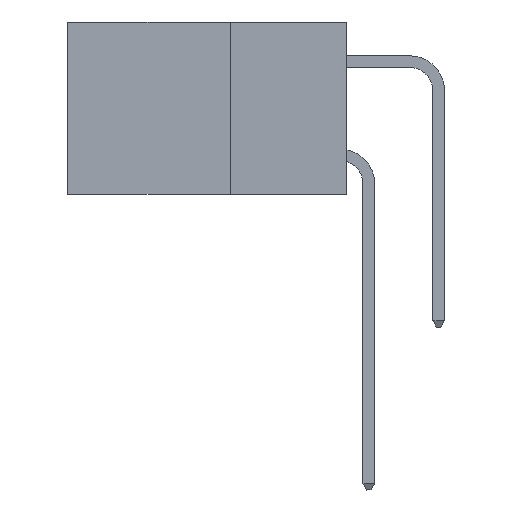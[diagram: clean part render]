
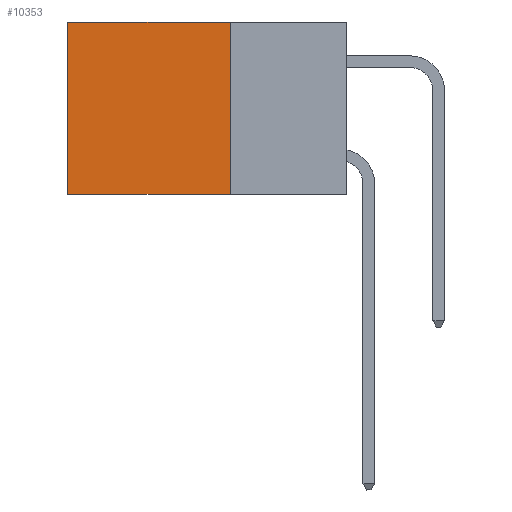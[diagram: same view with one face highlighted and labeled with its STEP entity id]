
A CAD part, left-side view. The second image highlights one B-rep face of the part: STEP entity #10353.
In plain terms, the highlighted planar face has unit normal (-1, 0, 0).
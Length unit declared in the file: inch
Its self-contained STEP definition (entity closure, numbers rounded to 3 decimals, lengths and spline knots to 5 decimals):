
#384 = LINE ( 'NONE', #24766, #29024 ) ;
#1726 = DIRECTION ( 'NONE',  ( 0., 1., 0. ) ) ;
#5333 = EDGE_CURVE ( 'NONE', #7010, #21526, #384, .T. ) ;
#6901 = CARTESIAN_POINT ( 'NONE',  ( 0.2875, 0.25, 0. ) ) ;
#7010 = VERTEX_POINT ( 'NONE', #28568 ) ;
#9095 = AXIS2_PLACEMENT_3D ( 'NONE', #33037, #10491, #24911 ) ;
#9684 = LINE ( 'NONE', #32237, #28303 ) ;
#10353 = ADVANCED_FACE ( 'NONE', ( #11183 ), #10658, .F. ) ;
#10491 = DIRECTION ( 'NONE',  ( 1., 0., 0. ) ) ;
#10658 = PLANE ( 'NONE',  #9095 ) ;
#11183 = FACE_OUTER_BOUND ( 'NONE', #15606, .T. ) ;
#12025 = CARTESIAN_POINT ( 'NONE',  ( 0.2875, 0.25, 0. ) ) ;
#12202 = CARTESIAN_POINT ( 'NONE',  ( 0.2875, 0.25, -0.37 ) ) ;
#12311 = DIRECTION ( 'NONE',  ( 0., 0., -1. ) ) ;
#12540 = VERTEX_POINT ( 'NONE', #12025 ) ;
#13928 = VERTEX_POINT ( 'NONE', #12202 ) ;
#14696 = VECTOR ( 'NONE', #12311, 39.37008 ) ;
#15580 = EDGE_CURVE ( 'NONE', #12540, #13928, #20804, .T. ) ;
#15606 = EDGE_LOOP ( 'NONE', ( #22739, #34669, #29979, #29397 ) ) ;
#17326 = VECTOR ( 'NONE', #19496, 39.37008 ) ;
#19496 = DIRECTION ( 'NONE',  ( 0., 1., 0. ) ) ;
#19716 = CARTESIAN_POINT ( 'NONE',  ( 0.2875, 0.6, -0.37 ) ) ;
#20804 = LINE ( 'NONE', #6901, #14696 ) ;
#21526 = VERTEX_POINT ( 'NONE', #19716 ) ;
#22054 = DIRECTION ( 'NONE',  ( 0., 0., -1. ) ) ;
#22739 = ORIENTED_EDGE ( 'NONE', *, *, #5333, .T. ) ;
#23210 = EDGE_CURVE ( 'NONE', #12540, #7010, #30872, .T. ) ;
#24766 = CARTESIAN_POINT ( 'NONE',  ( 0.2875, 0.6, 0. ) ) ;
#24911 = DIRECTION ( 'NONE',  ( 0., 0., -1. ) ) ;
#25100 = CARTESIAN_POINT ( 'NONE',  ( 0.2875, 0.25, 0. ) ) ;
#25356 = EDGE_CURVE ( 'NONE', #13928, #21526, #9684, .T. ) ;
#28303 = VECTOR ( 'NONE', #1726, 39.37008 ) ;
#28568 = CARTESIAN_POINT ( 'NONE',  ( 0.2875, 0.6, 0. ) ) ;
#29024 = VECTOR ( 'NONE', #22054, 39.37008 ) ;
#29397 = ORIENTED_EDGE ( 'NONE', *, *, #23210, .T. ) ;
#29979 = ORIENTED_EDGE ( 'NONE', *, *, #15580, .F. ) ;
#30872 = LINE ( 'NONE', #25100, #17326 ) ;
#32237 = CARTESIAN_POINT ( 'NONE',  ( 0.2875, 0.25, -0.37 ) ) ;
#33037 = CARTESIAN_POINT ( 'NONE',  ( 0.2875, 0.25, 0. ) ) ;
#34669 = ORIENTED_EDGE ( 'NONE', *, *, #25356, .F. ) ;
